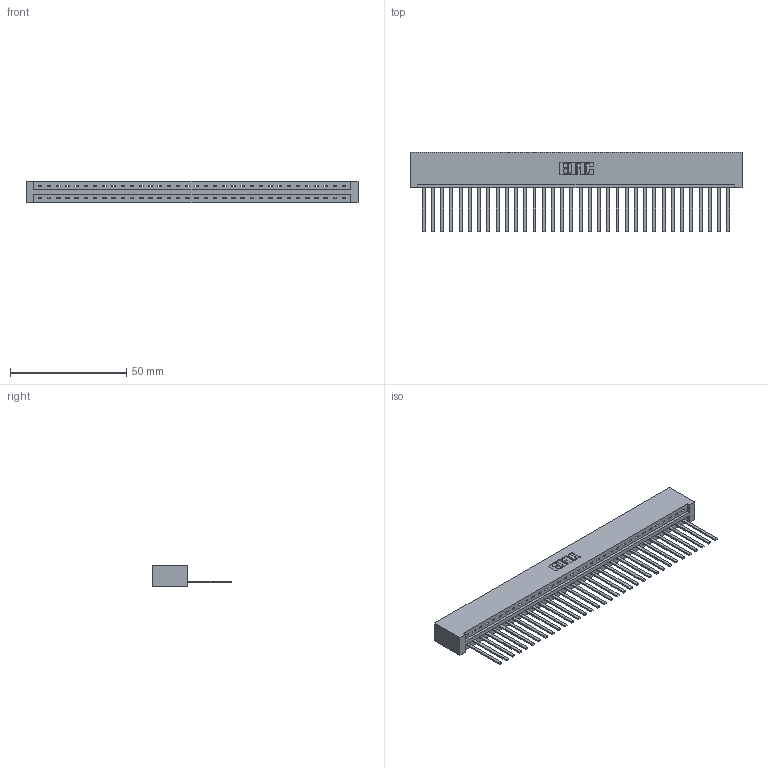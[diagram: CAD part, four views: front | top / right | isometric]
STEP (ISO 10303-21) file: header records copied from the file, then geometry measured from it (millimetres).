
FILE_DESCRIPTION (( 'STEP AP203' ), '1' );
FILE_NAME ('337-034-544-101.STEP', '2018-08-07T12:40:00', ( '' ), ( '' ), 'SwSTEP 2.0', 'SolidWorks 2016', '' );
FILE_SCHEMA (( 'CONFIG_CONTROL_DESIGN' ));
Length unit declared in the file: inch
Products named in the file (3): 337-034-544-101; 337 Part_No Mounting Lugs; 345-292-001_345-293-144
Assembly tree (35 placements, depth 2):
  337-034-544-101
    337 Part_No Mounting Lugs
    345-292-001_345-293-144  x34
Bounding box: 142.6 x 34.3 x 9.4 mm (x, y, z)
Volume: 15852.8 mm3; surface area: 17613.9 mm2
Topology: 35 solids, 35 shells, 2010 faces, 6067 edges, 3998 vertices
Faces by surface type: plane 1494, cylinder 516
Entity records: 25847 total; most frequent: CARTESIAN_POINT 4508, ORIENTED_EDGE 4478, DIRECTION 3799, EDGE_CURVE 2239, LINE 2123, VECTOR 2123, VERTEX_POINT 1490, AXIS2_PLACEMENT_3D 838
